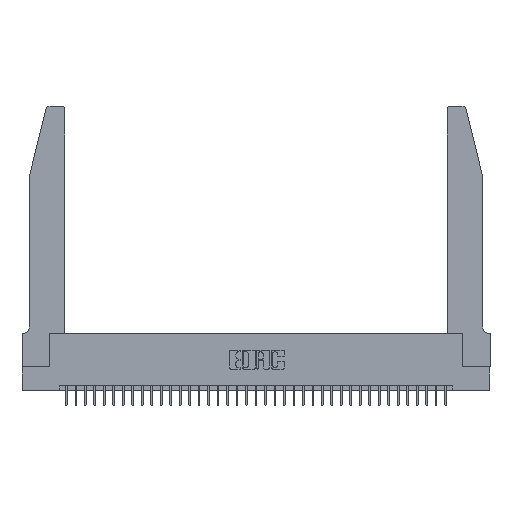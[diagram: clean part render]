
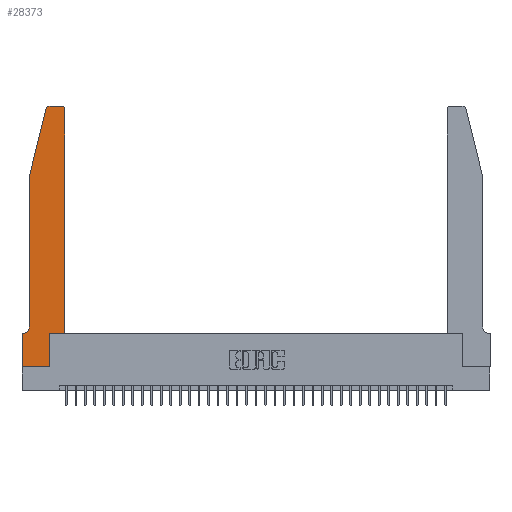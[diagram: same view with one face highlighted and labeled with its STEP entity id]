
A CAD part, top view. The second image highlights one B-rep face of the part: STEP entity #28373.
In plain terms, the highlighted planar face has unit normal (0, 0, 1).
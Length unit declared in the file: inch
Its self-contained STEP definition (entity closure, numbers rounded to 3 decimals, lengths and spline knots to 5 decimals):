
#117 = EDGE_LOOP ( 'NONE', ( #4993, #10376, #17618, #24835, #23161, #10649, #16232, #18004, #10499, #23439, #10629, #23336 ) ) ;
#708 = CARTESIAN_POINT ( 'NONE',  ( 0.0755, 2., 0.37 ) ) ;
#1145 = DIRECTION ( 'NONE',  ( -1., 0., 0. ) ) ;
#1156 = CARTESIAN_POINT ( 'NONE',  ( 0., 0., 0.37 ) ) ;
#2136 = VERTEX_POINT ( 'NONE', #18581 ) ;
#2355 = CARTESIAN_POINT ( 'NONE',  ( 0.284, 2.75, 0.37 ) ) ;
#3639 = DIRECTION ( 'NONE',  ( -0.239, -0.971, 0. ) ) ;
#3833 = EDGE_CURVE ( 'NONE', #27291, #14158, #24083, .T. ) ;
#3843 = AXIS2_PLACEMENT_3D ( 'NONE', #16193, #36110, #19056 ) ;
#4084 = DIRECTION ( 'NONE',  ( 0., -1., 0. ) ) ;
#4993 = ORIENTED_EDGE ( 'NONE', *, *, #25687, .T. ) ;
#5791 = CARTESIAN_POINT ( 'NONE',  ( 0., 0.35, 0.37 ) ) ;
#5973 = LINE ( 'NONE', #14676, #19475 ) ;
#6321 = VERTEX_POINT ( 'NONE', #31701 ) ;
#6407 = VERTEX_POINT ( 'NONE', #23571 ) ;
#6748 = CARTESIAN_POINT ( 'NONE',  ( 0.4205, 2.72, 0.37 ) ) ;
#7162 = AXIS2_PLACEMENT_3D ( 'NONE', #30251, #13187, #33100 ) ;
#7510 = VERTEX_POINT ( 'NONE', #5791 ) ;
#7536 = AXIS2_PLACEMENT_3D ( 'NONE', #6748, #26768, #9650 ) ;
#8573 = VECTOR ( 'NONE', #4084, 39.37008 ) ;
#8849 = DIRECTION ( 'NONE',  ( 1., 0., 0. ) ) ;
#9650 = DIRECTION ( 'NONE',  ( 1., 0., 0. ) ) ;
#9660 = EDGE_CURVE ( 'NONE', #14158, #2136, #17889, .T. ) ;
#10090 = VECTOR ( 'NONE', #8849, 39.37008 ) ;
#10376 = ORIENTED_EDGE ( 'NONE', *, *, #10853, .T. ) ;
#10499 = ORIENTED_EDGE ( 'NONE', *, *, #22111, .T. ) ;
#10629 = ORIENTED_EDGE ( 'NONE', *, *, #9660, .T. ) ;
#10649 = ORIENTED_EDGE ( 'NONE', *, *, #36874, .T. ) ;
#10853 = EDGE_CURVE ( 'NONE', #15983, #34605, #23098, .T. ) ;
#11239 = VERTEX_POINT ( 'NONE', #26329 ) ;
#11579 = VECTOR ( 'NONE', #3639, 39.37008 ) ;
#11968 = DIRECTION ( 'NONE',  ( 0., 0., -1. ) ) ;
#12033 = VECTOR ( 'NONE', #35925, 39.37008 ) ;
#12684 = LINE ( 'NONE', #16680, #19388 ) ;
#13063 = EDGE_CURVE ( 'NONE', #23189, #6321, #12684, .T. ) ;
#13187 = DIRECTION ( 'NONE',  ( 0., 0., 1. ) ) ;
#13727 = CARTESIAN_POINT ( 'NONE',  ( 0.0055, 0.35, 0.37 ) ) ;
#14158 = VERTEX_POINT ( 'NONE', #29078 ) ;
#14676 = CARTESIAN_POINT ( 'NONE',  ( 0.0755, 0.35, 0.37 ) ) ;
#14869 = DIRECTION ( 'NONE',  ( 1., 0., 0. ) ) ;
#15043 = EDGE_CURVE ( 'NONE', #7510, #27986, #31391, .T. ) ;
#15983 = VERTEX_POINT ( 'NONE', #2355 ) ;
#16193 = CARTESIAN_POINT ( 'NONE',  ( 0.284, 2.72, 0.37 ) ) ;
#16232 = ORIENTED_EDGE ( 'NONE', *, *, #15043, .T. ) ;
#16255 = AXIS2_PLACEMENT_3D ( 'NONE', #29051, #11968, #31907 ) ;
#16680 = CARTESIAN_POINT ( 'NONE',  ( 0.0755, 2., 0.37 ) ) ;
#17565 = DIRECTION ( 'NONE',  ( -1., 0., 0. ) ) ;
#17618 = ORIENTED_EDGE ( 'NONE', *, *, #21893, .T. ) ;
#17660 = LINE ( 'NONE', #35507, #32771 ) ;
#17889 = LINE ( 'NONE', #26699, #24513 ) ;
#18004 = ORIENTED_EDGE ( 'NONE', *, *, #23584, .T. ) ;
#18581 = CARTESIAN_POINT ( 'NONE',  ( 0.4505, 2.72, 0.37 ) ) ;
#19056 = DIRECTION ( 'NONE',  ( 1., 0., 0. ) ) ;
#19388 = VECTOR ( 'NONE', #33703, 39.37008 ) ;
#19475 = VECTOR ( 'NONE', #17565, 39.37008 ) ;
#21893 = EDGE_CURVE ( 'NONE', #34605, #23189, #26752, .T. ) ;
#22111 = EDGE_CURVE ( 'NONE', #6407, #27291, #27172, .T. ) ;
#22271 = FACE_OUTER_BOUND ( 'NONE', #117, .T. ) ;
#22387 = EDGE_CURVE ( 'NONE', #6321, #29760, #24919, .T. ) ;
#23098 = CIRCLE ( 'NONE', #3843, 0.03 ) ;
#23161 = ORIENTED_EDGE ( 'NONE', *, *, #22387, .T. ) ;
#23189 = VERTEX_POINT ( 'NONE', #32841 ) ;
#23336 = ORIENTED_EDGE ( 'NONE', *, *, #35845, .T. ) ;
#23439 = ORIENTED_EDGE ( 'NONE', *, *, #3833, .T. ) ;
#23571 = CARTESIAN_POINT ( 'NONE',  ( 0.2865, 0., 0.37 ) ) ;
#23584 = EDGE_CURVE ( 'NONE', #27986, #6407, #27074, .T. ) ;
#24083 = LINE ( 'NONE', #29056, #30811 ) ;
#24513 = VECTOR ( 'NONE', #29589, 39.37008 ) ;
#24835 = ORIENTED_EDGE ( 'NONE', *, *, #13063, .T. ) ;
#24870 = CIRCLE ( 'NONE', #7536, 0.03 ) ;
#24919 = CIRCLE ( 'NONE', #16255, 0.07 ) ;
#25687 = EDGE_CURVE ( 'NONE', #11239, #15983, #17660, .T. ) ;
#26329 = CARTESIAN_POINT ( 'NONE',  ( 0.4205, 2.75, 0.37 ) ) ;
#26699 = CARTESIAN_POINT ( 'NONE',  ( 0.4505, 0.35, 0.37 ) ) ;
#26752 = LINE ( 'NONE', #708, #11579 ) ;
#26768 = DIRECTION ( 'NONE',  ( 0., 0., 1. ) ) ;
#27074 = LINE ( 'NONE', #28850, #10090 ) ;
#27172 = LINE ( 'NONE', #33154, #12033 ) ;
#27291 = VERTEX_POINT ( 'NONE', #27896 ) ;
#27896 = CARTESIAN_POINT ( 'NONE',  ( 0.2865, 0.35, 0.37 ) ) ;
#27986 = VERTEX_POINT ( 'NONE', #31116 ) ;
#28373 = ADVANCED_FACE ( 'NONE', ( #22271 ), #35873, .T. ) ;
#28850 = CARTESIAN_POINT ( 'NONE',  ( 0., 0., 0.37 ) ) ;
#29051 = CARTESIAN_POINT ( 'NONE',  ( 0.0055, 0.42, 0.37 ) ) ;
#29056 = CARTESIAN_POINT ( 'NONE',  ( 0.4505, 0.35, 0.37 ) ) ;
#29078 = CARTESIAN_POINT ( 'NONE',  ( 0.4505, 0.35, 0.37 ) ) ;
#29589 = DIRECTION ( 'NONE',  ( 0., 1., 0. ) ) ;
#29760 = VERTEX_POINT ( 'NONE', #13727 ) ;
#30251 = CARTESIAN_POINT ( 'NONE',  ( 0., 0.35, 0.37 ) ) ;
#30811 = VECTOR ( 'NONE', #14869, 39.37008 ) ;
#31116 = CARTESIAN_POINT ( 'NONE',  ( 0., 0., 0.37 ) ) ;
#31391 = LINE ( 'NONE', #1156, #8573 ) ;
#31701 = CARTESIAN_POINT ( 'NONE',  ( 0.0755, 0.42, 0.37 ) ) ;
#31907 = DIRECTION ( 'NONE',  ( -1., 0., 0. ) ) ;
#32771 = VECTOR ( 'NONE', #1145, 39.37008 ) ;
#32841 = CARTESIAN_POINT ( 'NONE',  ( 0.0755, 2., 0.37 ) ) ;
#33100 = DIRECTION ( 'NONE',  ( 1., 0., 0. ) ) ;
#33154 = CARTESIAN_POINT ( 'NONE',  ( 0.2865, 0.35, 0.37 ) ) ;
#33703 = DIRECTION ( 'NONE',  ( 0., -1., 0. ) ) ;
#34605 = VERTEX_POINT ( 'NONE', #35361 ) ;
#35361 = CARTESIAN_POINT ( 'NONE',  ( 0.25487, 2.72718, 0.37 ) ) ;
#35507 = CARTESIAN_POINT ( 'NONE',  ( 0.2605, 2.75, 0.37 ) ) ;
#35845 = EDGE_CURVE ( 'NONE', #2136, #11239, #24870, .T. ) ;
#35873 = PLANE ( 'NONE',  #7162 ) ;
#35925 = DIRECTION ( 'NONE',  ( 0., 1., 0. ) ) ;
#36110 = DIRECTION ( 'NONE',  ( 0., 0., 1. ) ) ;
#36874 = EDGE_CURVE ( 'NONE', #29760, #7510, #5973, .T. ) ;
